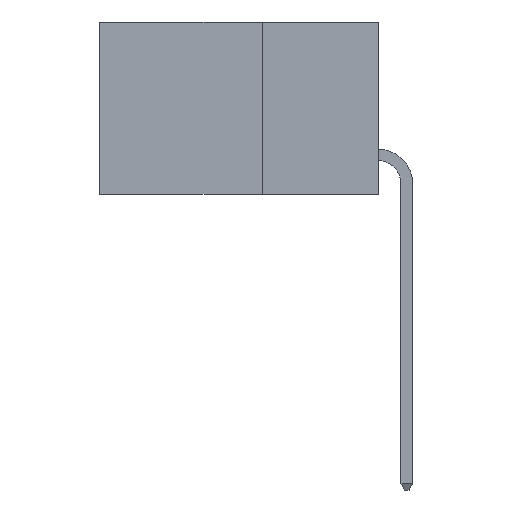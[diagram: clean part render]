
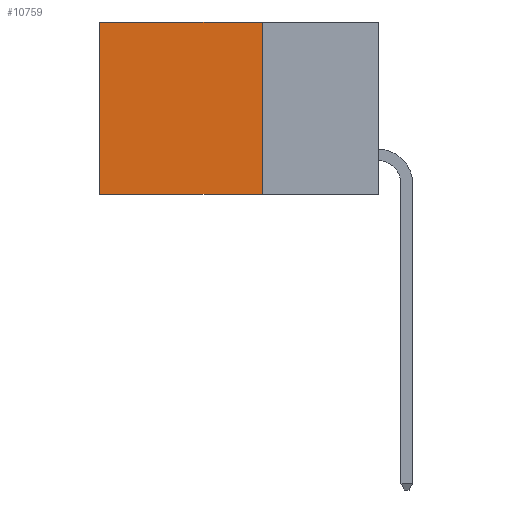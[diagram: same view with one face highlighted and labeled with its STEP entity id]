
A CAD part, left-side view. The second image highlights one B-rep face of the part: STEP entity #10759.
In plain terms, the highlighted planar face has unit normal (-1, 0, 0).
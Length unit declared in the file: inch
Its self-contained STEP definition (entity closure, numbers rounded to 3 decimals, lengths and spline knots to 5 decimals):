
#149 = CARTESIAN_POINT ( 'NONE',  ( 0.2615, 0.6, -0.37 ) ) ;
#1573 = AXIS2_PLACEMENT_3D ( 'NONE', #21409, #21081, #21072 ) ;
#2571 = VECTOR ( 'NONE', #18012, 39.37008 ) ;
#3199 = LINE ( 'NONE', #20920, #2571 ) ;
#3883 = DIRECTION ( 'NONE',  ( 0., 0., -1. ) ) ;
#4133 = EDGE_CURVE ( 'NONE', #22245, #6764, #8655, .T. ) ;
#6764 = VERTEX_POINT ( 'NONE', #17550 ) ;
#7551 = VERTEX_POINT ( 'NONE', #8656 ) ;
#8066 = VECTOR ( 'NONE', #24254, 39.37008 ) ;
#8506 = EDGE_CURVE ( 'NONE', #15489, #22245, #3199, .T. ) ;
#8655 = LINE ( 'NONE', #149, #8066 ) ;
#8656 = CARTESIAN_POINT ( 'NONE',  ( 0.2615, 0.25, -0.37 ) ) ;
#9541 = VECTOR ( 'NONE', #3883, 39.37008 ) ;
#10126 = LINE ( 'NONE', #13386, #9541 ) ;
#10759 = ADVANCED_FACE ( 'NONE', ( #15244 ), #21099, .F. ) ;
#11052 = ORIENTED_EDGE ( 'NONE', *, *, #11123, .F. ) ;
#11123 = EDGE_CURVE ( 'NONE', #7551, #6764, #23225, .T. ) ;
#11279 = ORIENTED_EDGE ( 'NONE', *, *, #21244, .F. ) ;
#11639 = CARTESIAN_POINT ( 'NONE',  ( 0.2615, 0.25, 0. ) ) ;
#13386 = CARTESIAN_POINT ( 'NONE',  ( 0.2615, 0.25, -0.37 ) ) ;
#15244 = FACE_OUTER_BOUND ( 'NONE', #20668, .T. ) ;
#15489 = VERTEX_POINT ( 'NONE', #11639 ) ;
#16498 = ORIENTED_EDGE ( 'NONE', *, *, #8506, .T. ) ;
#17116 = DIRECTION ( 'NONE',  ( 0., 1., 0. ) ) ;
#17137 = CARTESIAN_POINT ( 'NONE',  ( 0.2615, 0.25, -0.37 ) ) ;
#17550 = CARTESIAN_POINT ( 'NONE',  ( 0.2615, 0.6, -0.37 ) ) ;
#18012 = DIRECTION ( 'NONE',  ( 0., 1., 0. ) ) ;
#18667 = ORIENTED_EDGE ( 'NONE', *, *, #4133, .T. ) ;
#20668 = EDGE_LOOP ( 'NONE', ( #18667, #11052, #11279, #16498 ) ) ;
#20920 = CARTESIAN_POINT ( 'NONE',  ( 0.2615, 0.25, 0. ) ) ;
#21072 = DIRECTION ( 'NONE',  ( 0., 0., -1. ) ) ;
#21081 = DIRECTION ( 'NONE',  ( 1., 0., 0. ) ) ;
#21099 = PLANE ( 'NONE',  #1573 ) ;
#21244 = EDGE_CURVE ( 'NONE', #15489, #7551, #10126, .T. ) ;
#21409 = CARTESIAN_POINT ( 'NONE',  ( 0.2615, 0.25, -0.37 ) ) ;
#22245 = VERTEX_POINT ( 'NONE', #22959 ) ;
#22959 = CARTESIAN_POINT ( 'NONE',  ( 0.2615, 0.6, 0. ) ) ;
#23225 = LINE ( 'NONE', #17137, #23797 ) ;
#23797 = VECTOR ( 'NONE', #17116, 39.37008 ) ;
#24254 = DIRECTION ( 'NONE',  ( 0., 0., -1. ) ) ;
